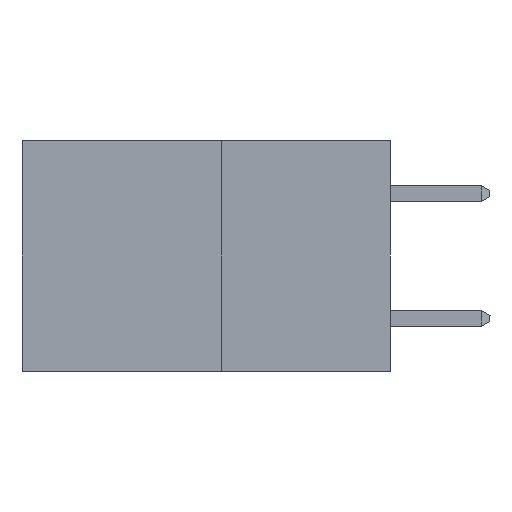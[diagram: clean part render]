
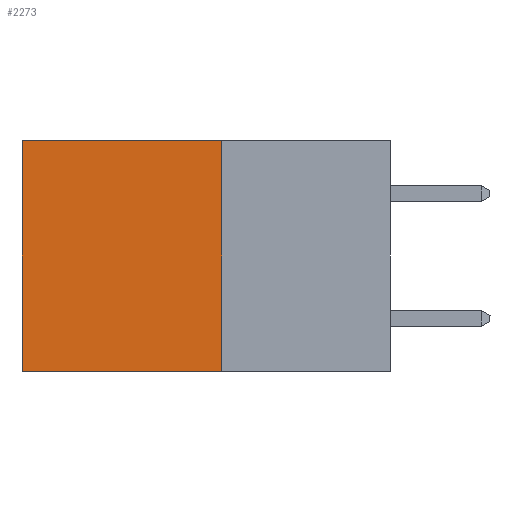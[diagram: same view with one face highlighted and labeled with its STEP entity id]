
A CAD part, left-side view. The second image highlights one B-rep face of the part: STEP entity #2273.
In plain terms, the highlighted planar face has unit normal (-1, 0, 0).
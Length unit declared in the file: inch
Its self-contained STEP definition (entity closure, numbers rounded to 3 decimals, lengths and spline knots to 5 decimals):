
#130 = CARTESIAN_POINT ( 'NONE',  ( 0.277, 0.59, -0.37 ) ) ;
#401 = VERTEX_POINT ( 'NONE', #4071 ) ;
#2273 = ADVANCED_FACE ( 'NONE', ( #10339 ), #4242, .F. ) ;
#2293 = CARTESIAN_POINT ( 'NONE',  ( 0.277, 0.27, -0.37 ) ) ;
#2571 = EDGE_LOOP ( 'NONE', ( #3126, #7877, #3408, #5788 ) ) ;
#2572 = EDGE_CURVE ( 'NONE', #401, #8334, #4086, .T. ) ;
#2633 = DIRECTION ( 'NONE',  ( 1., 0., 0. ) ) ;
#2742 = VECTOR ( 'NONE', #6474, 39.37008 ) ;
#3126 = ORIENTED_EDGE ( 'NONE', *, *, #7660, .T. ) ;
#3283 = LINE ( 'NONE', #6522, #2742 ) ;
#3408 = ORIENTED_EDGE ( 'NONE', *, *, #5748, .F. ) ;
#3880 = DIRECTION ( 'NONE',  ( 0., 1., 0. ) ) ;
#4071 = CARTESIAN_POINT ( 'NONE',  ( 0.277, 0.27, -0.37 ) ) ;
#4086 = LINE ( 'NONE', #10504, #6444 ) ;
#4242 = PLANE ( 'NONE',  #7504 ) ;
#4510 = CARTESIAN_POINT ( 'NONE',  ( 0.277, 0.27, 0. ) ) ;
#4714 = CARTESIAN_POINT ( 'NONE',  ( 0.277, 0.27, -0.37 ) ) ;
#4768 = DIRECTION ( 'NONE',  ( 0., 0., -1. ) ) ;
#4924 = CARTESIAN_POINT ( 'NONE',  ( 0.277, 0.27, 0. ) ) ;
#5285 = VECTOR ( 'NONE', #4768, 39.37008 ) ;
#5748 = EDGE_CURVE ( 'NONE', #8734, #401, #7363, .T. ) ;
#5788 = ORIENTED_EDGE ( 'NONE', *, *, #8460, .T. ) ;
#6444 = VECTOR ( 'NONE', #3880, 39.37008 ) ;
#6474 = DIRECTION ( 'NONE',  ( 0., 0., -1. ) ) ;
#6522 = CARTESIAN_POINT ( 'NONE',  ( 0.277, 0.59, -0.37 ) ) ;
#7070 = DIRECTION ( 'NONE',  ( 0., 0., -1. ) ) ;
#7363 = LINE ( 'NONE', #4714, #5285 ) ;
#7504 = AXIS2_PLACEMENT_3D ( 'NONE', #2293, #2633, #7070 ) ;
#7660 = EDGE_CURVE ( 'NONE', #11452, #8334, #3283, .T. ) ;
#7877 = ORIENTED_EDGE ( 'NONE', *, *, #2572, .F. ) ;
#8129 = LINE ( 'NONE', #4924, #10448 ) ;
#8334 = VERTEX_POINT ( 'NONE', #130 ) ;
#8460 = EDGE_CURVE ( 'NONE', #8734, #11452, #8129, .T. ) ;
#8734 = VERTEX_POINT ( 'NONE', #4510 ) ;
#9338 = DIRECTION ( 'NONE',  ( 0., 1., 0. ) ) ;
#10134 = CARTESIAN_POINT ( 'NONE',  ( 0.277, 0.59, 0. ) ) ;
#10339 = FACE_OUTER_BOUND ( 'NONE', #2571, .T. ) ;
#10448 = VECTOR ( 'NONE', #9338, 39.37008 ) ;
#10504 = CARTESIAN_POINT ( 'NONE',  ( 0.277, 0.27, -0.37 ) ) ;
#11452 = VERTEX_POINT ( 'NONE', #10134 ) ;
